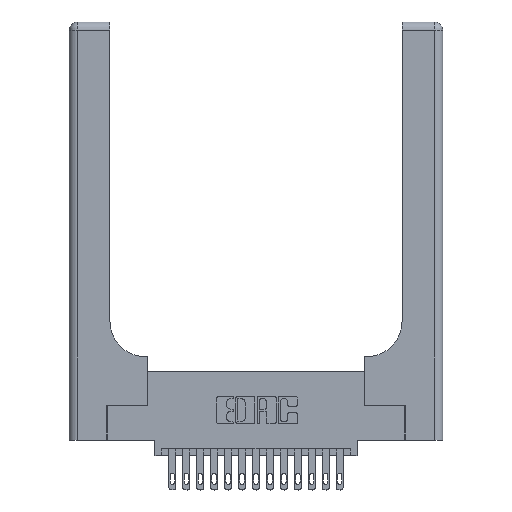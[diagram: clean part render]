
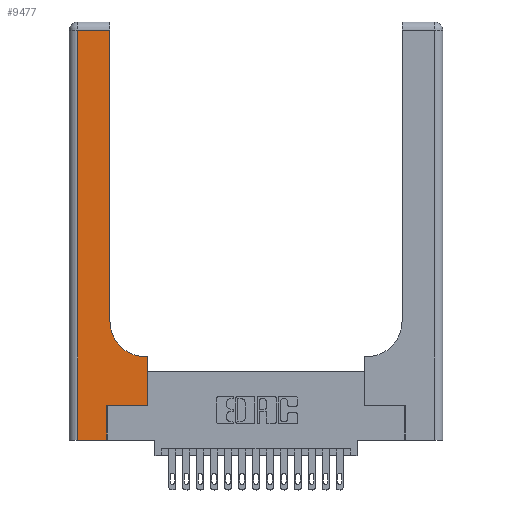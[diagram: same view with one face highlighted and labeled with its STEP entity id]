
A CAD part, top view. The second image highlights one B-rep face of the part: STEP entity #9477.
In plain terms, the highlighted planar face has unit normal (0, 0, 1).
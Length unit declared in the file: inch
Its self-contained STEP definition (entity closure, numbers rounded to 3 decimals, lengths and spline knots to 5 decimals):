
#333 = DIRECTION ( 'NONE',  ( -1., 0., 0. ) ) ;
#533 = VERTEX_POINT ( 'NONE', #7011 ) ;
#677 = VERTEX_POINT ( 'NONE', #18034 ) ;
#679 = ORIENTED_EDGE ( 'NONE', *, *, #12136, .T. ) ;
#1222 = CARTESIAN_POINT ( 'NONE',  ( 0., 2.94, 0.37 ) ) ;
#1658 = DIRECTION ( 'NONE',  ( 0., 0., -1. ) ) ;
#1664 = VECTOR ( 'NONE', #17539, 39.37008 ) ;
#1927 = VECTOR ( 'NONE', #8309, 39.37008 ) ;
#1956 = AXIS2_PLACEMENT_3D ( 'NONE', #16003, #10147, #7030 ) ;
#2390 = CARTESIAN_POINT ( 'NONE',  ( 0.2915, 3., 0.37 ) ) ;
#2456 = CARTESIAN_POINT ( 'NONE',  ( 0.06, 2.94, 0.37 ) ) ;
#2514 = CARTESIAN_POINT ( 'NONE',  ( 0.269, 0.25, 0.37 ) ) ;
#2717 = DIRECTION ( 'NONE',  ( -1., 0., 0. ) ) ;
#2761 = CARTESIAN_POINT ( 'NONE',  ( 0.06, 0., 0.37 ) ) ;
#3213 = ORIENTED_EDGE ( 'NONE', *, *, #16344, .T. ) ;
#3233 = ORIENTED_EDGE ( 'NONE', *, *, #18886, .T. ) ;
#3281 = CARTESIAN_POINT ( 'NONE',  ( 0., 3., 0.37 ) ) ;
#3288 = EDGE_CURVE ( 'NONE', #677, #15763, #12441, .T. ) ;
#3696 = EDGE_CURVE ( 'NONE', #12581, #16511, #6334, .T. ) ;
#3886 = EDGE_LOOP ( 'NONE', ( #16996, #679, #5233, #3233, #16762, #9832, #3213, #19091, #7863 ) ) ;
#3915 = VECTOR ( 'NONE', #18560, 39.37008 ) ;
#4618 = LINE ( 'NONE', #4708, #16325 ) ;
#4655 = CARTESIAN_POINT ( 'NONE',  ( 0.2915, 2.94, 0.37 ) ) ;
#4708 = CARTESIAN_POINT ( 'NONE',  ( 0.06, 3., 0.37 ) ) ;
#4915 = DIRECTION ( 'NONE',  ( -1., 0., 0. ) ) ;
#5233 = ORIENTED_EDGE ( 'NONE', *, *, #14603, .T. ) ;
#5239 = CARTESIAN_POINT ( 'NONE',  ( 0.269, 0., 0.37 ) ) ;
#5716 = LINE ( 'NONE', #18453, #17228 ) ;
#5966 = LINE ( 'NONE', #12188, #14187 ) ;
#6075 = VERTEX_POINT ( 'NONE', #18270 ) ;
#6319 = CARTESIAN_POINT ( 'NONE',  ( 0.269, 0.25, 0.37 ) ) ;
#6334 = LINE ( 'NONE', #6319, #9141 ) ;
#6686 = FACE_OUTER_BOUND ( 'NONE', #3886, .T. ) ;
#7011 = CARTESIAN_POINT ( 'NONE',  ( 0.269, 0., 0.37 ) ) ;
#7030 = DIRECTION ( 'NONE',  ( 1., 0., 0. ) ) ;
#7045 = CARTESIAN_POINT ( 'NONE',  ( 0., 0., 0.37 ) ) ;
#7863 = ORIENTED_EDGE ( 'NONE', *, *, #3288, .T. ) ;
#8309 = DIRECTION ( 'NONE',  ( 0., 1., 0. ) ) ;
#8773 = VERTEX_POINT ( 'NONE', #2456 ) ;
#9141 = VECTOR ( 'NONE', #16826, 39.37008 ) ;
#9477 = ADVANCED_FACE ( 'NONE', ( #6686 ), #15277, .F. ) ;
#9537 = VERTEX_POINT ( 'NONE', #4655 ) ;
#9832 = ORIENTED_EDGE ( 'NONE', *, *, #3696, .T. ) ;
#9859 = LINE ( 'NONE', #5239, #1927 ) ;
#9969 = EDGE_CURVE ( 'NONE', #6075, #677, #5966, .T. ) ;
#10147 = DIRECTION ( 'NONE',  ( 0., 0., -1. ) ) ;
#12136 = EDGE_CURVE ( 'NONE', #9537, #8773, #12228, .T. ) ;
#12188 = CARTESIAN_POINT ( 'NONE',  ( 0.2915, 0.6, 0.37 ) ) ;
#12228 = LINE ( 'NONE', #1222, #17436 ) ;
#12441 = CIRCLE ( 'NONE', #1956, 0.25 ) ;
#12510 = EDGE_CURVE ( 'NONE', #533, #12581, #9859, .T. ) ;
#12581 = VERTEX_POINT ( 'NONE', #2514 ) ;
#12677 = VERTEX_POINT ( 'NONE', #2761 ) ;
#14187 = VECTOR ( 'NONE', #333, 39.37008 ) ;
#14385 = CARTESIAN_POINT ( 'NONE',  ( 0.5585, 0.25, 0.37 ) ) ;
#14603 = EDGE_CURVE ( 'NONE', #8773, #12677, #4618, .T. ) ;
#15249 = LINE ( 'NONE', #7045, #1664 ) ;
#15257 = DIRECTION ( 'NONE',  ( 0., -1., 0. ) ) ;
#15272 = EDGE_CURVE ( 'NONE', #15763, #9537, #15625, .T. ) ;
#15277 = PLANE ( 'NONE',  #15575 ) ;
#15575 = AXIS2_PLACEMENT_3D ( 'NONE', #3281, #1658, #4915 ) ;
#15625 = LINE ( 'NONE', #2390, #3915 ) ;
#15763 = VERTEX_POINT ( 'NONE', #18343 ) ;
#16003 = CARTESIAN_POINT ( 'NONE',  ( 0.5415, 0.85, 0.37 ) ) ;
#16325 = VECTOR ( 'NONE', #15257, 39.37008 ) ;
#16344 = EDGE_CURVE ( 'NONE', #16511, #6075, #5716, .T. ) ;
#16511 = VERTEX_POINT ( 'NONE', #14385 ) ;
#16762 = ORIENTED_EDGE ( 'NONE', *, *, #12510, .T. ) ;
#16826 = DIRECTION ( 'NONE',  ( 1., 0., 0. ) ) ;
#16996 = ORIENTED_EDGE ( 'NONE', *, *, #15272, .T. ) ;
#17019 = DIRECTION ( 'NONE',  ( 0., 1., 0. ) ) ;
#17228 = VECTOR ( 'NONE', #17019, 39.37008 ) ;
#17436 = VECTOR ( 'NONE', #2717, 39.37008 ) ;
#17539 = DIRECTION ( 'NONE',  ( 1., 0., 0. ) ) ;
#18034 = CARTESIAN_POINT ( 'NONE',  ( 0.5415, 0.6, 0.37 ) ) ;
#18270 = CARTESIAN_POINT ( 'NONE',  ( 0.5585, 0.6, 0.37 ) ) ;
#18343 = CARTESIAN_POINT ( 'NONE',  ( 0.2915, 0.85, 0.37 ) ) ;
#18453 = CARTESIAN_POINT ( 'NONE',  ( 0.5585, 0.25, 0.37 ) ) ;
#18560 = DIRECTION ( 'NONE',  ( 0., 1., 0. ) ) ;
#18886 = EDGE_CURVE ( 'NONE', #12677, #533, #15249, .T. ) ;
#19091 = ORIENTED_EDGE ( 'NONE', *, *, #9969, .T. ) ;
